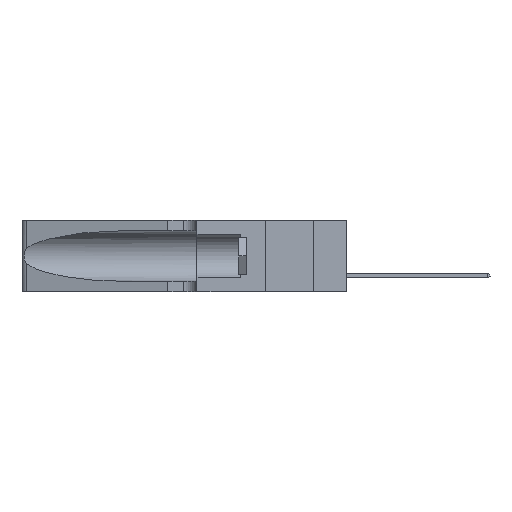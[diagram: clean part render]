
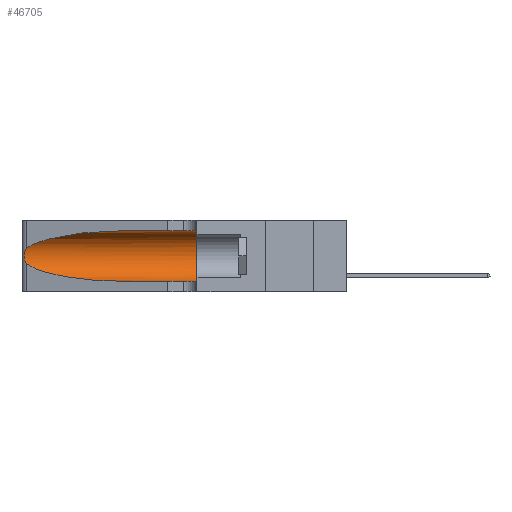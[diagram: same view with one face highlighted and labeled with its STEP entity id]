
A CAD part, left-side view. The second image highlights one B-rep face of the part: STEP entity #46705.
In plain terms, the highlighted cylindrical face has radius 3.308 mm (diameter 6.617 mm), a partial arc.
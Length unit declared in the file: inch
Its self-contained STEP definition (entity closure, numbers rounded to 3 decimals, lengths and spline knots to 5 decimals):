
#4017 = CARTESIAN_POINT ( 'NONE',  ( 0.1305, 1.61858, 0.31525 ) ) ;
#5029 = EDGE_CURVE ( 'NONE', #49377, #15573, #37379, .T. ) ;
#5077 =( BOUNDED_CURVE ( )  B_SPLINE_CURVE ( 3, ( #10712, #19031, #32448, #20070 ),
 .UNSPECIFIED., .F., .F. ) 
 B_SPLINE_CURVE_WITH_KNOTS ( ( 4, 4 ),
 ( 3.44316, 4.71239 ),
 .UNSPECIFIED. ) 
 CURVE ( )  GEOMETRIC_REPRESENTATION_ITEM ( )  RATIONAL_B_SPLINE_CURVE ( ( 1., 0.87, 0.87, 1. ) ) 
 REPRESENTATION_ITEM ( '' )  );
#5132 = VECTOR ( 'NONE', #16442, 39.37008 ) ;
#6594 = AXIS2_PLACEMENT_3D ( 'NONE', #13589, #21394, #29526 ) ;
#7102 = CARTESIAN_POINT ( 'NONE',  ( 0.1305, 0.72297, 0.31525 ) ) ;
#8154 = EDGE_CURVE ( 'NONE', #32502, #44173, #5077, .T. ) ;
#8659 = CYLINDRICAL_SURFACE ( 'NONE', #35068, 0.13025 ) ;
#8817 = CARTESIAN_POINT ( 'NONE',  ( 0.25854, 1.2359, 0.20912 ) ) ;
#8968 = CARTESIAN_POINT ( 'NONE',  ( 0.1305, 0.35, 0.05475 ) ) ;
#9834 = LINE ( 'NONE', #4017, #30753 ) ;
#10359 = ORIENTED_EDGE ( 'NONE', *, *, #8154, .T. ) ;
#10712 = CARTESIAN_POINT ( 'NONE',  ( 0.25487, 1.22718, 0.14631 ) ) ;
#11093 = CARTESIAN_POINT ( 'NONE',  ( 0.25487, 1.22718, 0.14631 ) ) ;
#11377 = ORIENTED_EDGE ( 'NONE', *, *, #23318, .T. ) ;
#11872 = ORIENTED_EDGE ( 'NONE', *, *, #38152, .T. ) ;
#12893 = CARTESIAN_POINT ( 'NONE',  ( 0.25856, 1.23593, 0.16098 ) ) ;
#13050 = CARTESIAN_POINT ( 'NONE',  ( 0.25789, 1.23486, 0.15765 ) ) ;
#13450 = CARTESIAN_POINT ( 'NONE',  ( 0.1305, 0.72297, 0.31525 ) ) ;
#13589 = CARTESIAN_POINT ( 'NONE',  ( 0.1305, 0.35, 0.185 ) ) ;
#14148 = CARTESIAN_POINT ( 'NONE',  ( 0.1305, 1.61858, 0.185 ) ) ;
#15573 = VERTEX_POINT ( 'NONE', #8968 ) ;
#16442 = DIRECTION ( 'NONE',  ( 0., -1., 0. ) ) ;
#17020 =( BOUNDED_CURVE ( )  B_SPLINE_CURVE ( 3, ( #7102, #20522, #37004, #28823 ),
 .UNSPECIFIED., .F., .F. ) 
 B_SPLINE_CURVE_WITH_KNOTS ( ( 4, 4 ),
 ( 1.5708, 2.84003 ),
 .UNSPECIFIED. ) 
 CURVE ( )  GEOMETRIC_REPRESENTATION_ITEM ( )  RATIONAL_B_SPLINE_CURVE ( ( 1., 0.87, 0.87, 1. ) ) 
 REPRESENTATION_ITEM ( '' )  );
#17997 = CARTESIAN_POINT ( 'NONE',  ( 0.25639, 1.23186, 0.15144 ) ) ;
#19031 = CARTESIAN_POINT ( 'NONE',  ( 0.2373, 1.15595, 0.08982 ) ) ;
#20070 = CARTESIAN_POINT ( 'NONE',  ( 0.1305, 0.72297, 0.05475 ) ) ;
#20522 = CARTESIAN_POINT ( 'NONE',  ( 0.18966, 0.96281, 0.31525 ) ) ;
#21241 = CARTESIAN_POINT ( 'NONE',  ( 0.1305, 1.61858, 0.05475 ) ) ;
#21394 = DIRECTION ( 'NONE',  ( 0., 1., 0. ) ) ;
#22416 = VERTEX_POINT ( 'NONE', #22574 ) ;
#22574 = CARTESIAN_POINT ( 'NONE',  ( 0.25487, 1.22718, 0.22369 ) ) ;
#23318 = EDGE_CURVE ( 'NONE', #31097, #22416, #17020, .T. ) ;
#24729 = CARTESIAN_POINT ( 'NONE',  ( 0.26075, 1.23896, 0.19203 ) ) ;
#28130 = EDGE_LOOP ( 'NONE', ( #11377, #39977, #10359, #11872, #41342, #45845 ) ) ;
#28805 = CARTESIAN_POINT ( 'NONE',  ( 0.26075, 1.23896, 0.178 ) ) ;
#28823 = CARTESIAN_POINT ( 'NONE',  ( 0.25487, 1.22718, 0.22369 ) ) ;
#29526 = DIRECTION ( 'NONE',  ( 0., 0., 1. ) ) ;
#30188 = FACE_OUTER_BOUND ( 'NONE', #28130, .T. ) ;
#30753 = VECTOR ( 'NONE', #36047, 39.37008 ) ;
#31097 = VERTEX_POINT ( 'NONE', #13450 ) ;
#32448 = CARTESIAN_POINT ( 'NONE',  ( 0.18966, 0.96281, 0.05475 ) ) ;
#32502 = VERTEX_POINT ( 'NONE', #11093 ) ;
#33066 = CARTESIAN_POINT ( 'NONE',  ( 0.25639, 1.23184, 0.21858 ) ) ;
#33956 = CARTESIAN_POINT ( 'NONE',  ( 0.25555, 1.22993, 0.14849 ) ) ;
#34285 = LINE ( 'NONE', #21241, #5132 ) ;
#35068 = AXIS2_PLACEMENT_3D ( 'NONE', #14148, #50658, #51167 ) ;
#36047 = DIRECTION ( 'NONE',  ( 0., -1., 0. ) ) ;
#37004 = CARTESIAN_POINT ( 'NONE',  ( 0.2373, 1.15595, 0.28018 ) ) ;
#37151 = CARTESIAN_POINT ( 'NONE',  ( 0.26017, 1.23833, 0.17102 ) ) ;
#37379 = CIRCLE ( 'NONE', #6594, 0.13025 ) ;
#38054 = CARTESIAN_POINT ( 'NONE',  ( 0.25487, 1.22718, 0.14631 ) ) ;
#38152 = EDGE_CURVE ( 'NONE', #44173, #15573, #34285, .T. ) ;
#39977 = ORIENTED_EDGE ( 'NONE', *, *, #51502, .T. ) ;
#41051 = CARTESIAN_POINT ( 'NONE',  ( 0.25555, 1.22994, 0.2215 ) ) ;
#41342 = ORIENTED_EDGE ( 'NONE', *, *, #5029, .F. ) ;
#41744 = CARTESIAN_POINT ( 'NONE',  ( 0.25787, 1.23484, 0.2124 ) ) ;
#42691 = CARTESIAN_POINT ( 'NONE',  ( 0.1305, 0.35, 0.31525 ) ) ;
#44173 = VERTEX_POINT ( 'NONE', #45430 ) ;
#45430 = CARTESIAN_POINT ( 'NONE',  ( 0.1305, 0.72297, 0.05475 ) ) ;
#45677 = CARTESIAN_POINT ( 'NONE',  ( 0.25487, 1.22718, 0.22369 ) ) ;
#45845 = ORIENTED_EDGE ( 'NONE', *, *, #47403, .F. ) ;
#45854 = CARTESIAN_POINT ( 'NONE',  ( 0.26018, 1.23835, 0.19895 ) ) ;
#46705 = ADVANCED_FACE ( 'NONE', ( #30188 ), #8659, .F. ) ;
#47403 = EDGE_CURVE ( 'NONE', #31097, #49377, #9834, .T. ) ;
#49377 = VERTEX_POINT ( 'NONE', #42691 ) ;
#49871 = B_SPLINE_CURVE_WITH_KNOTS ( 'NONE', 3,
 ( #45677, #41051, #33066, #41744, #8817, #45854, #24729, #28805, #37151, #12893, #13050, #17997, #33956, #38054 ),
 .UNSPECIFIED., .F., .F.,
 ( 4, 2, 2, 2, 2, 2, 4 ),
 ( 0., 0.00027, 0.00053, 0.00107, 0.0016, 0.00187, 0.00214 ),
 .UNSPECIFIED. ) ;
#50658 = DIRECTION ( 'NONE',  ( 0., -1., 0. ) ) ;
#51167 = DIRECTION ( 'NONE',  ( 0., 0., -1. ) ) ;
#51502 = EDGE_CURVE ( 'NONE', #22416, #32502, #49871, .T. ) ;
